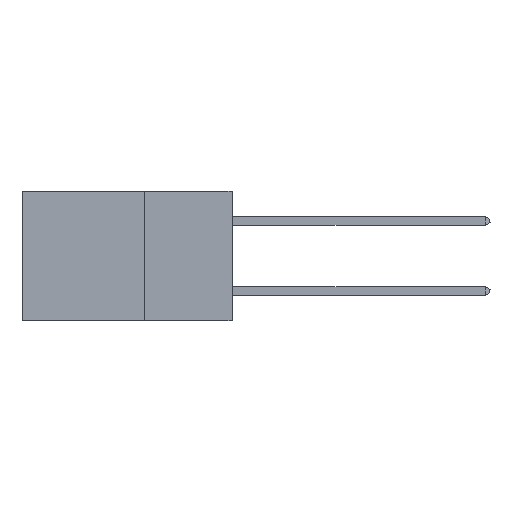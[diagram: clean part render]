
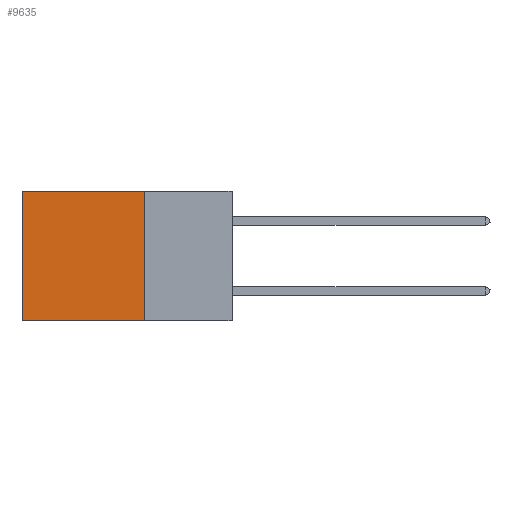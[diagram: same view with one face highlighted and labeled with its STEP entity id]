
A CAD part, left-side view. The second image highlights one B-rep face of the part: STEP entity #9635.
In plain terms, the highlighted planar face has unit normal (-1, 0, 0).
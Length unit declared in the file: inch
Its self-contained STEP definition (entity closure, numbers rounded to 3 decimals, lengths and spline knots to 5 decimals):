
#200 = VERTEX_POINT ( 'NONE', #8360 ) ;
#439 = ORIENTED_EDGE ( 'NONE', *, *, #29114, .T. ) ;
#1236 = EDGE_CURVE ( 'NONE', #7561, #200, #11146, .T. ) ;
#1378 = ORIENTED_EDGE ( 'NONE', *, *, #24790, .T. ) ;
#5911 = CARTESIAN_POINT ( 'NONE',  ( 0.2875, 0.25, -0.37 ) ) ;
#5990 = CARTESIAN_POINT ( 'NONE',  ( 0.2875, 0.25, 0. ) ) ;
#7561 = VERTEX_POINT ( 'NONE', #5990 ) ;
#8360 = CARTESIAN_POINT ( 'NONE',  ( 0.2875, 0.25, -0.37 ) ) ;
#9635 = ADVANCED_FACE ( 'NONE', ( #19600 ), #29663, .F. ) ;
#9913 = LINE ( 'NONE', #14743, #33803 ) ;
#11146 = LINE ( 'NONE', #17633, #30073 ) ;
#12470 = DIRECTION ( 'NONE',  ( 0., 0., -1. ) ) ;
#13825 = DIRECTION ( 'NONE',  ( 1., 0., 0. ) ) ;
#14635 = DIRECTION ( 'NONE',  ( 0., 1., 0. ) ) ;
#14743 = CARTESIAN_POINT ( 'NONE',  ( 0.2875, 0.6, 0. ) ) ;
#14841 = LINE ( 'NONE', #18065, #15261 ) ;
#15261 = VECTOR ( 'NONE', #20607, 39.37008 ) ;
#17633 = CARTESIAN_POINT ( 'NONE',  ( 0.2875, 0.25, 0. ) ) ;
#17717 = DIRECTION ( 'NONE',  ( 0., 0., -1. ) ) ;
#17887 = CARTESIAN_POINT ( 'NONE',  ( 0.2875, 0.6, 0. ) ) ;
#18065 = CARTESIAN_POINT ( 'NONE',  ( 0.2875, 0.25, 0. ) ) ;
#19600 = FACE_OUTER_BOUND ( 'NONE', #23880, .T. ) ;
#20607 = DIRECTION ( 'NONE',  ( 0., 1., 0. ) ) ;
#21241 = VECTOR ( 'NONE', #14635, 39.37008 ) ;
#21940 = ORIENTED_EDGE ( 'NONE', *, *, #22171, .F. ) ;
#22171 = EDGE_CURVE ( 'NONE', #200, #31920, #27356, .T. ) ;
#22422 = CARTESIAN_POINT ( 'NONE',  ( 0.2875, 0.6, -0.37 ) ) ;
#23476 = ORIENTED_EDGE ( 'NONE', *, *, #1236, .F. ) ;
#23880 = EDGE_LOOP ( 'NONE', ( #1378, #21940, #23476, #439 ) ) ;
#24155 = AXIS2_PLACEMENT_3D ( 'NONE', #26872, #13825, #32235 ) ;
#24790 = EDGE_CURVE ( 'NONE', #30447, #31920, #9913, .T. ) ;
#26872 = CARTESIAN_POINT ( 'NONE',  ( 0.2875, 0.25, 0. ) ) ;
#27356 = LINE ( 'NONE', #5911, #21241 ) ;
#29114 = EDGE_CURVE ( 'NONE', #7561, #30447, #14841, .T. ) ;
#29663 = PLANE ( 'NONE',  #24155 ) ;
#30073 = VECTOR ( 'NONE', #12470, 39.37008 ) ;
#30447 = VERTEX_POINT ( 'NONE', #17887 ) ;
#31920 = VERTEX_POINT ( 'NONE', #22422 ) ;
#32235 = DIRECTION ( 'NONE',  ( 0., 0., -1. ) ) ;
#33803 = VECTOR ( 'NONE', #17717, 39.37008 ) ;
